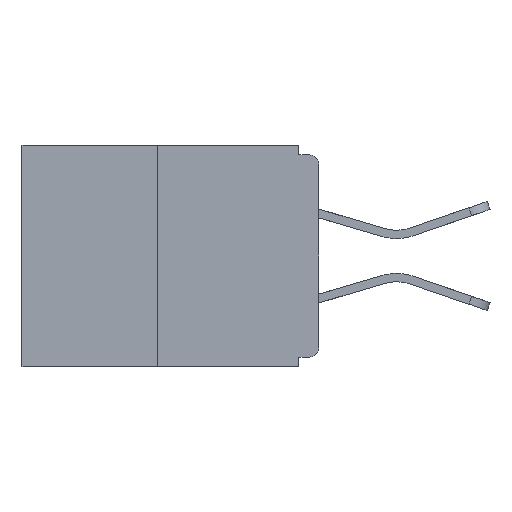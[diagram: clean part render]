
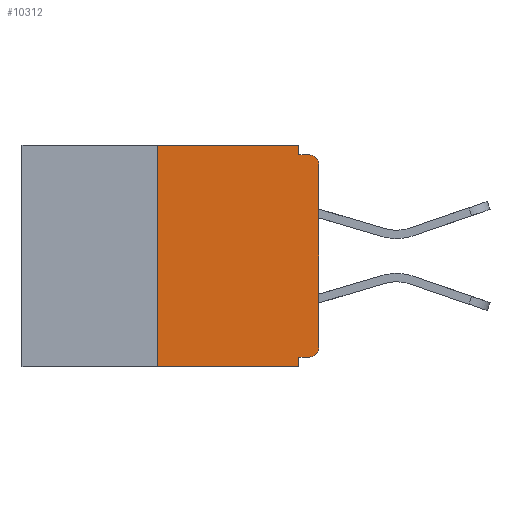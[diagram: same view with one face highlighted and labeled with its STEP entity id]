
A CAD part, left-side view. The second image highlights one B-rep face of the part: STEP entity #10312.
In plain terms, the highlighted planar face has unit normal (-1, 0, 0).
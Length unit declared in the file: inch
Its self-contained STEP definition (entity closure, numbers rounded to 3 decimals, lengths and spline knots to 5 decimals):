
#246 = EDGE_CURVE ( 'NONE', #2809, #12458, #10391, .T. ) ;
#408 = EDGE_CURVE ( 'NONE', #3593, #18271, #15878, .T. ) ;
#433 = CARTESIAN_POINT ( 'NONE',  ( 0., 0.031, 0. ) ) ;
#776 = LINE ( 'NONE', #7169, #2012 ) ;
#985 = CARTESIAN_POINT ( 'NONE',  ( 0., 0.46, -0.343 ) ) ;
#1267 = DIRECTION ( 'NONE',  ( -1., 0., 0. ) ) ;
#1366 = DIRECTION ( 'NONE',  ( 0., 0., -1. ) ) ;
#1771 = VERTEX_POINT ( 'NONE', #1881 ) ;
#1834 = ORIENTED_EDGE ( 'NONE', *, *, #5664, .F. ) ;
#1881 = CARTESIAN_POINT ( 'NONE',  ( 0., 0.25, -0.343 ) ) ;
#1907 = AXIS2_PLACEMENT_3D ( 'NONE', #15770, #12340, #1366 ) ;
#2012 = VECTOR ( 'NONE', #13508, 39.37008 ) ;
#2154 = CARTESIAN_POINT ( 'NONE',  ( 0., 0.031, -0.343 ) ) ;
#2282 = ORIENTED_EDGE ( 'NONE', *, *, #408, .F. ) ;
#2752 = ORIENTED_EDGE ( 'NONE', *, *, #2881, .T. ) ;
#2807 = VERTEX_POINT ( 'NONE', #4790 ) ;
#2809 = VERTEX_POINT ( 'NONE', #15977 ) ;
#2862 = AXIS2_PLACEMENT_3D ( 'NONE', #4649, #14179, #3097 ) ;
#2881 = EDGE_CURVE ( 'NONE', #18170, #19635, #10266, .T. ) ;
#3012 = CIRCLE ( 'NONE', #20321, 0.015 ) ;
#3088 = VECTOR ( 'NONE', #16458, 39.37008 ) ;
#3097 = DIRECTION ( 'NONE',  ( 0., 0., -1. ) ) ;
#3593 = VERTEX_POINT ( 'NONE', #15527 ) ;
#3624 = DIRECTION ( 'NONE',  ( 0., 0., 1. ) ) ;
#4649 = CARTESIAN_POINT ( 'NONE',  ( 0., 0.46, 0. ) ) ;
#4686 = DIRECTION ( 'NONE',  ( 0., 1., 0. ) ) ;
#4790 = CARTESIAN_POINT ( 'NONE',  ( 0., 0.031, -0.015 ) ) ;
#5281 = LINE ( 'NONE', #11583, #6250 ) ;
#5625 = EDGE_CURVE ( 'NONE', #1771, #15606, #15293, .T. ) ;
#5664 = EDGE_CURVE ( 'NONE', #12458, #2807, #776, .T. ) ;
#6250 = VECTOR ( 'NONE', #3624, 39.37008 ) ;
#6375 = EDGE_CURVE ( 'NONE', #1771, #2809, #5281, .T. ) ;
#6675 = LINE ( 'NONE', #2154, #3088 ) ;
#6849 = CARTESIAN_POINT ( 'NONE',  ( 0., 0., -0.015 ) ) ;
#7169 = CARTESIAN_POINT ( 'NONE',  ( 0., 0.031, 0. ) ) ;
#7237 = VERTEX_POINT ( 'NONE', #18879 ) ;
#7663 = DIRECTION ( 'NONE',  ( 0., 0., -1. ) ) ;
#7835 = PLANE ( 'NONE',  #2862 ) ;
#8534 = DIRECTION ( 'NONE',  ( 0., -1., 0. ) ) ;
#8561 = ORIENTED_EDGE ( 'NONE', *, *, #6375, .F. ) ;
#8755 = ORIENTED_EDGE ( 'NONE', *, *, #11448, .T. ) ;
#8836 = VECTOR ( 'NONE', #9852, 39.37008 ) ;
#9019 = CARTESIAN_POINT ( 'NONE',  ( 0., 0.015, -0.313 ) ) ;
#9598 = ORIENTED_EDGE ( 'NONE', *, *, #16784, .F. ) ;
#9604 = CIRCLE ( 'NONE', #1907, 0.015 ) ;
#9852 = DIRECTION ( 'NONE',  ( 0., 0., 1. ) ) ;
#10266 = LINE ( 'NONE', #14811, #8836 ) ;
#10312 = ADVANCED_FACE ( 'NONE', ( #15844 ), #7835, .F. ) ;
#10391 = LINE ( 'NONE', #18163, #13594 ) ;
#11448 = EDGE_CURVE ( 'NONE', #19635, #7237, #9604, .T. ) ;
#11583 = CARTESIAN_POINT ( 'NONE',  ( 0., 0.25, 0. ) ) ;
#12340 = DIRECTION ( 'NONE',  ( -1., 0., 0. ) ) ;
#12458 = VERTEX_POINT ( 'NONE', #433 ) ;
#12671 = ORIENTED_EDGE ( 'NONE', *, *, #5625, .T. ) ;
#13075 = LINE ( 'NONE', #6849, #14388 ) ;
#13508 = DIRECTION ( 'NONE',  ( 0., 0., -1. ) ) ;
#13594 = VECTOR ( 'NONE', #18590, 39.37008 ) ;
#13721 = DIRECTION ( 'NONE',  ( 0., -1., 0. ) ) ;
#14179 = DIRECTION ( 'NONE',  ( 1., 0., 0. ) ) ;
#14388 = VECTOR ( 'NONE', #8534, 39.37008 ) ;
#14811 = CARTESIAN_POINT ( 'NONE',  ( 0., 0., 0. ) ) ;
#15293 = LINE ( 'NONE', #985, #15707 ) ;
#15527 = CARTESIAN_POINT ( 'NONE',  ( 0., 0.015, -0.328 ) ) ;
#15549 = EDGE_CURVE ( 'NONE', #3593, #18170, #3012, .T. ) ;
#15606 = VERTEX_POINT ( 'NONE', #17325 ) ;
#15707 = VECTOR ( 'NONE', #13721, 39.37008 ) ;
#15770 = CARTESIAN_POINT ( 'NONE',  ( 0., 0.015, -0.03 ) ) ;
#15844 = FACE_OUTER_BOUND ( 'NONE', #18529, .T. ) ;
#15878 = LINE ( 'NONE', #19001, #18539 ) ;
#15977 = CARTESIAN_POINT ( 'NONE',  ( 0., 0.25, 0. ) ) ;
#16107 = CARTESIAN_POINT ( 'NONE',  ( 0., 0.031, -0.328 ) ) ;
#16458 = DIRECTION ( 'NONE',  ( 0., 0., -1. ) ) ;
#16784 = EDGE_CURVE ( 'NONE', #2807, #7237, #13075, .T. ) ;
#17325 = CARTESIAN_POINT ( 'NONE',  ( 0., 0.031, -0.343 ) ) ;
#18040 = EDGE_CURVE ( 'NONE', #18271, #15606, #6675, .T. ) ;
#18163 = CARTESIAN_POINT ( 'NONE',  ( 0., 0.46, 0. ) ) ;
#18170 = VERTEX_POINT ( 'NONE', #18621 ) ;
#18271 = VERTEX_POINT ( 'NONE', #16107 ) ;
#18529 = EDGE_LOOP ( 'NONE', ( #18662, #8561, #12671, #19488, #2282, #19492, #2752, #8755, #9598, #1834 ) ) ;
#18539 = VECTOR ( 'NONE', #4686, 39.37008 ) ;
#18590 = DIRECTION ( 'NONE',  ( 0., -1., 0. ) ) ;
#18621 = CARTESIAN_POINT ( 'NONE',  ( 0., 0., -0.313 ) ) ;
#18662 = ORIENTED_EDGE ( 'NONE', *, *, #246, .F. ) ;
#18879 = CARTESIAN_POINT ( 'NONE',  ( 0., 0.015, -0.015 ) ) ;
#19001 = CARTESIAN_POINT ( 'NONE',  ( 0., 0., -0.328 ) ) ;
#19488 = ORIENTED_EDGE ( 'NONE', *, *, #18040, .F. ) ;
#19492 = ORIENTED_EDGE ( 'NONE', *, *, #15549, .T. ) ;
#19635 = VERTEX_POINT ( 'NONE', #20359 ) ;
#20321 = AXIS2_PLACEMENT_3D ( 'NONE', #9019, #1267, #7663 ) ;
#20359 = CARTESIAN_POINT ( 'NONE',  ( 0., 0., -0.03 ) ) ;
